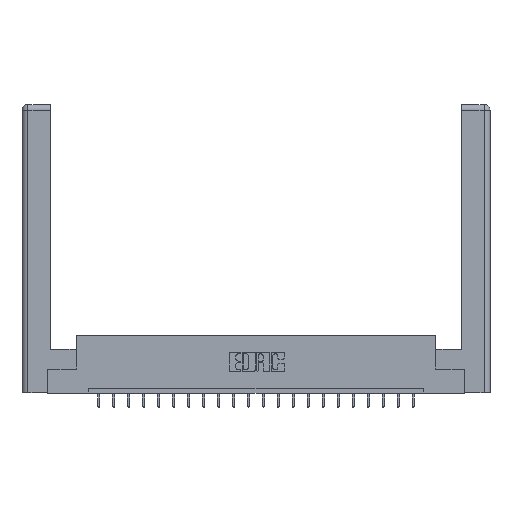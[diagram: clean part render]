
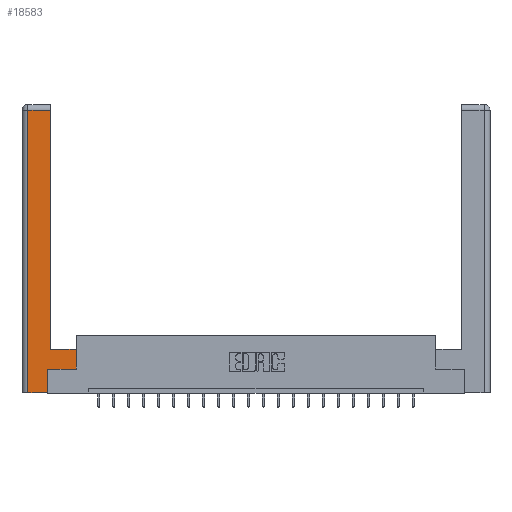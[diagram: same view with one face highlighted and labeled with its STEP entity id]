
A CAD part, top view. The second image highlights one B-rep face of the part: STEP entity #18583.
In plain terms, the highlighted planar face has unit normal (0, 0, 1).
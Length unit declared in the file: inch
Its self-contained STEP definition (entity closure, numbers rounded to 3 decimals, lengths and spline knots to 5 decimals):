
#738 = ORIENTED_EDGE ( 'NONE', *, *, #5503, .T. ) ;
#1241 = EDGE_CURVE ( 'NONE', #10193, #6262, #10168, .T. ) ;
#1258 = DIRECTION ( 'NONE',  ( -1., 0., 0. ) ) ;
#1368 = DIRECTION ( 'NONE',  ( 0., -1., 0. ) ) ;
#1493 = CARTESIAN_POINT ( 'NONE',  ( 0.0615, 0., 0. ) ) ;
#1773 = LINE ( 'NONE', #11991, #9564 ) ;
#2484 = CARTESIAN_POINT ( 'NONE',  ( 0.295, 2.94, 0. ) ) ;
#2568 = LINE ( 'NONE', #14304, #14283 ) ;
#2926 = CARTESIAN_POINT ( 'NONE',  ( 0.265, 0.245, 0. ) ) ;
#3118 = ORIENTED_EDGE ( 'NONE', *, *, #8990, .T. ) ;
#3222 = VERTEX_POINT ( 'NONE', #1493 ) ;
#3267 = CARTESIAN_POINT ( 'NONE',  ( 0.295, 0.45, 0. ) ) ;
#3522 = CARTESIAN_POINT ( 'NONE',  ( 0.565, 0.245, 0. ) ) ;
#4004 = VECTOR ( 'NONE', #7962, 39.37008 ) ;
#4480 = VECTOR ( 'NONE', #17392, 39.37008 ) ;
#4594 = PLANE ( 'NONE',  #13106 ) ;
#4877 = CARTESIAN_POINT ( 'NONE',  ( 0.0615, 2.94, 0. ) ) ;
#5275 = DIRECTION ( 'NONE',  ( 0., 1., 0. ) ) ;
#5503 = EDGE_CURVE ( 'NONE', #19682, #13111, #12848, .T. ) ;
#6095 = CARTESIAN_POINT ( 'NONE',  ( 0.265, 0., 0. ) ) ;
#6262 = VERTEX_POINT ( 'NONE', #10568 ) ;
#6402 = VERTEX_POINT ( 'NONE', #19567 ) ;
#6433 = EDGE_CURVE ( 'NONE', #6262, #3222, #8085, .T. ) ;
#6702 = EDGE_CURVE ( 'NONE', #13172, #11556, #8858, .T. ) ;
#7573 = LINE ( 'NONE', #10838, #9152 ) ;
#7619 = DIRECTION ( 'NONE',  ( 0., 1., 0. ) ) ;
#7733 = DIRECTION ( 'NONE',  ( -1., 0., 0. ) ) ;
#7803 = EDGE_CURVE ( 'NONE', #11556, #10193, #2568, .T. ) ;
#7962 = DIRECTION ( 'NONE',  ( 1., 0., 0. ) ) ;
#8085 = LINE ( 'NONE', #11362, #20870 ) ;
#8858 = LINE ( 'NONE', #12368, #18503 ) ;
#8990 = EDGE_CURVE ( 'NONE', #3222, #6402, #12865, .T. ) ;
#9152 = VECTOR ( 'NONE', #7619, 39.37008 ) ;
#9564 = VECTOR ( 'NONE', #5275, 39.37008 ) ;
#9618 = ORIENTED_EDGE ( 'NONE', *, *, #13654, .T. ) ;
#10168 = LINE ( 'NONE', #4877, #18741 ) ;
#10193 = VERTEX_POINT ( 'NONE', #2484 ) ;
#10568 = CARTESIAN_POINT ( 'NONE',  ( 0.0615, 2.94, 0. ) ) ;
#10838 = CARTESIAN_POINT ( 'NONE',  ( 0.265, 0.245, 0. ) ) ;
#11108 = DIRECTION ( 'NONE',  ( 0., 1., 0. ) ) ;
#11120 = ORIENTED_EDGE ( 'NONE', *, *, #6433, .T. ) ;
#11249 = EDGE_CURVE ( 'NONE', #6402, #19682, #7573, .T. ) ;
#11322 = DIRECTION ( 'NONE',  ( 0., 0., -1. ) ) ;
#11362 = CARTESIAN_POINT ( 'NONE',  ( 0.0615, 0., 0. ) ) ;
#11556 = VERTEX_POINT ( 'NONE', #3267 ) ;
#11991 = CARTESIAN_POINT ( 'NONE',  ( 0.565, 0.45, 0. ) ) ;
#12368 = CARTESIAN_POINT ( 'NONE',  ( 0.295, 0.45, 0. ) ) ;
#12848 = LINE ( 'NONE', #14053, #4480 ) ;
#12865 = LINE ( 'NONE', #6095, #4004 ) ;
#13106 = AXIS2_PLACEMENT_3D ( 'NONE', #19461, #11322, #7733 ) ;
#13111 = VERTEX_POINT ( 'NONE', #3522 ) ;
#13172 = VERTEX_POINT ( 'NONE', #20346 ) ;
#13654 = EDGE_CURVE ( 'NONE', #13111, #13172, #1773, .T. ) ;
#13736 = ORIENTED_EDGE ( 'NONE', *, *, #6702, .T. ) ;
#14053 = CARTESIAN_POINT ( 'NONE',  ( 0.565, 0.245, 0. ) ) ;
#14283 = VECTOR ( 'NONE', #11108, 39.37008 ) ;
#14304 = CARTESIAN_POINT ( 'NONE',  ( 0.295, 3., 0. ) ) ;
#15896 = ORIENTED_EDGE ( 'NONE', *, *, #11249, .T. ) ;
#16600 = FACE_OUTER_BOUND ( 'NONE', #18811, .T. ) ;
#17392 = DIRECTION ( 'NONE',  ( 1., 0., 0. ) ) ;
#17841 = DIRECTION ( 'NONE',  ( -1., 0., 0. ) ) ;
#18503 = VECTOR ( 'NONE', #1258, 39.37008 ) ;
#18583 = ADVANCED_FACE ( 'NONE', ( #16600 ), #4594, .F. ) ;
#18741 = VECTOR ( 'NONE', #17841, 39.37008 ) ;
#18811 = EDGE_LOOP ( 'NONE', ( #18877, #19584, #11120, #3118, #15896, #738, #9618, #13736 ) ) ;
#18877 = ORIENTED_EDGE ( 'NONE', *, *, #7803, .T. ) ;
#19461 = CARTESIAN_POINT ( 'NONE',  ( 0., 0., 0. ) ) ;
#19567 = CARTESIAN_POINT ( 'NONE',  ( 0.265, 0., 0. ) ) ;
#19584 = ORIENTED_EDGE ( 'NONE', *, *, #1241, .T. ) ;
#19682 = VERTEX_POINT ( 'NONE', #2926 ) ;
#20346 = CARTESIAN_POINT ( 'NONE',  ( 0.565, 0.45, 0. ) ) ;
#20870 = VECTOR ( 'NONE', #1368, 39.37008 ) ;
